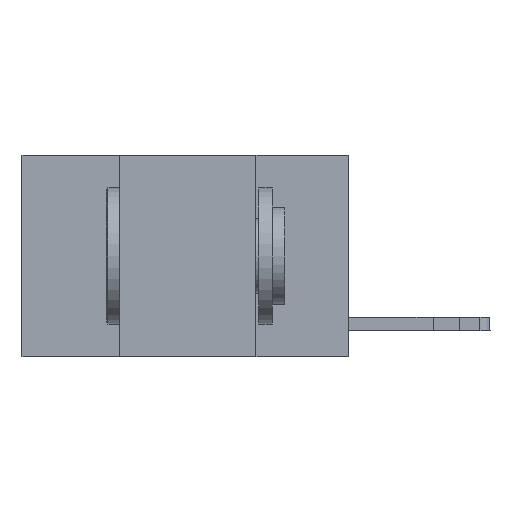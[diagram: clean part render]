
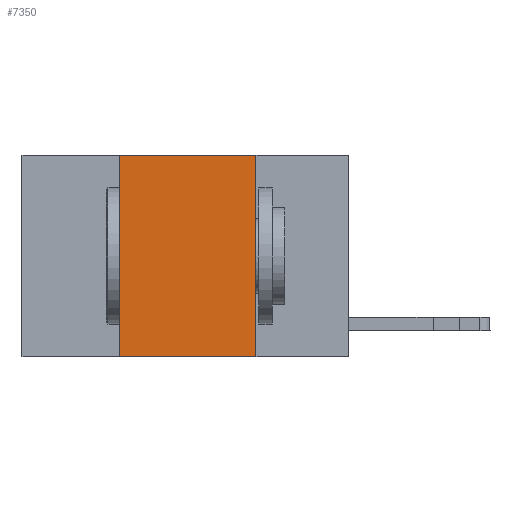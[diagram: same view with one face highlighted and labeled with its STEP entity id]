
A CAD part, left-side view. The second image highlights one B-rep face of the part: STEP entity #7350.
In plain terms, the highlighted planar face has unit normal (-1, 0, 0).
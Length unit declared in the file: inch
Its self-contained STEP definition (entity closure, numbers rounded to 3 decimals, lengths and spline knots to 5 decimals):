
#67 = VERTEX_POINT ( 'NONE', #12304 ) ;
#96 = ORIENTED_EDGE ( 'NONE', *, *, #9307, .F. ) ;
#282 = CARTESIAN_POINT ( 'NONE',  ( 0., 0.17, -0.37 ) ) ;
#330 = PLANE ( 'NONE',  #11661 ) ;
#442 = ORIENTED_EDGE ( 'NONE', *, *, #2009, .F. ) ;
#494 = ORIENTED_EDGE ( 'NONE', *, *, #9549, .T. ) ;
#1183 = FACE_OUTER_BOUND ( 'NONE', #12461, .T. ) ;
#1975 = VECTOR ( 'NONE', #10017, 39.37008 ) ;
#2009 = EDGE_CURVE ( 'NONE', #67, #4840, #4628, .T. ) ;
#3356 = LINE ( 'NONE', #6582, #5750 ) ;
#3459 = VERTEX_POINT ( 'NONE', #282 ) ;
#3820 = VECTOR ( 'NONE', #5110, 39.37008 ) ;
#4081 = CARTESIAN_POINT ( 'NONE',  ( 0., 0.6, 0. ) ) ;
#4519 = DIRECTION ( 'NONE',  ( 0., -1., 0. ) ) ;
#4628 = LINE ( 'NONE', #6924, #1975 ) ;
#4840 = VERTEX_POINT ( 'NONE', #9442 ) ;
#5110 = DIRECTION ( 'NONE',  ( 0., -1., 0. ) ) ;
#5547 = CARTESIAN_POINT ( 'NONE',  ( 0., 0.17, 0. ) ) ;
#5750 = VECTOR ( 'NONE', #4519, 39.37008 ) ;
#6582 = CARTESIAN_POINT ( 'NONE',  ( 0., 0.6, -0.37 ) ) ;
#6924 = CARTESIAN_POINT ( 'NONE',  ( 0., 0.42, 0. ) ) ;
#7192 = VECTOR ( 'NONE', #12609, 39.37008 ) ;
#7350 = ADVANCED_FACE ( 'NONE', ( #1183 ), #330, .F. ) ;
#9307 = EDGE_CURVE ( 'NONE', #4840, #10379, #12046, .T. ) ;
#9442 = CARTESIAN_POINT ( 'NONE',  ( 0., 0.42, 0. ) ) ;
#9549 = EDGE_CURVE ( 'NONE', #67, #3459, #3356, .T. ) ;
#9999 = LINE ( 'NONE', #11674, #7192 ) ;
#10017 = DIRECTION ( 'NONE',  ( 0., 0., 1. ) ) ;
#10379 = VERTEX_POINT ( 'NONE', #5547 ) ;
#11661 = AXIS2_PLACEMENT_3D ( 'NONE', #13171, #13164, #13161 ) ;
#11674 = CARTESIAN_POINT ( 'NONE',  ( 0., 0.17, 0. ) ) ;
#12046 = LINE ( 'NONE', #4081, #3820 ) ;
#12304 = CARTESIAN_POINT ( 'NONE',  ( 0., 0.42, -0.37 ) ) ;
#12461 = EDGE_LOOP ( 'NONE', ( #12807, #96, #442, #494 ) ) ;
#12609 = DIRECTION ( 'NONE',  ( 0., 0., -1. ) ) ;
#12676 = EDGE_CURVE ( 'NONE', #10379, #3459, #9999, .T. ) ;
#12807 = ORIENTED_EDGE ( 'NONE', *, *, #12676, .F. ) ;
#13161 = DIRECTION ( 'NONE',  ( 0., 0., -1. ) ) ;
#13164 = DIRECTION ( 'NONE',  ( 1., 0., 0. ) ) ;
#13171 = CARTESIAN_POINT ( 'NONE',  ( 0., 0.6, 0. ) ) ;
